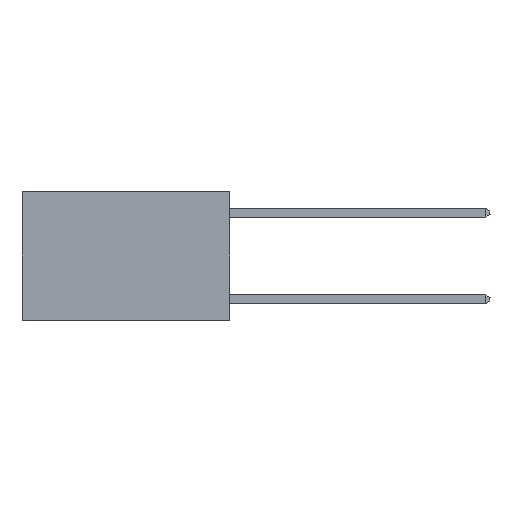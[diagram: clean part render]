
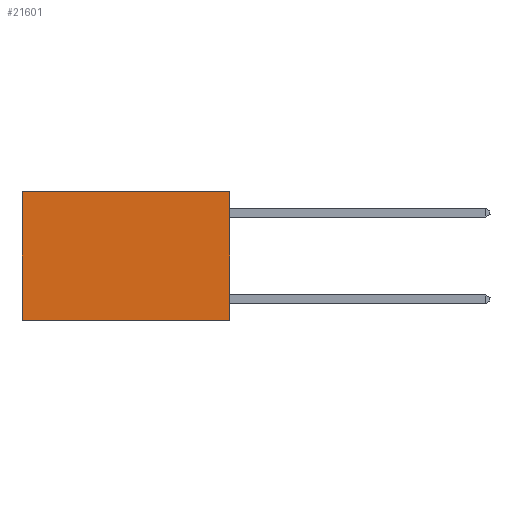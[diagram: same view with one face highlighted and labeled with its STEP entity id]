
A CAD part, left-side view. The second image highlights one B-rep face of the part: STEP entity #21601.
In plain terms, the highlighted planar face has unit normal (-1, 0, 0).
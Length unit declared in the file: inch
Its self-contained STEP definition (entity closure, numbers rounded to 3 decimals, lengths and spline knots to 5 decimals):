
#163 = VECTOR ( 'NONE', #21086, 39.37008 ) ;
#412 = ORIENTED_EDGE ( 'NONE', *, *, #11139, .T. ) ;
#1876 = EDGE_LOOP ( 'NONE', ( #2396, #12379, #10127, #412 ) ) ;
#2396 = ORIENTED_EDGE ( 'NONE', *, *, #17601, .T. ) ;
#2932 = LINE ( 'NONE', #8210, #163 ) ;
#3527 = CARTESIAN_POINT ( 'NONE',  ( 0.2625, 0., 0. ) ) ;
#5244 = CARTESIAN_POINT ( 'NONE',  ( 0.2625, 0., 0. ) ) ;
#5309 = CARTESIAN_POINT ( 'NONE',  ( 0.2625, 0.6, -0.37 ) ) ;
#5475 = PLANE ( 'NONE',  #11655 ) ;
#5821 = VERTEX_POINT ( 'NONE', #9431 ) ;
#8210 = CARTESIAN_POINT ( 'NONE',  ( 0.2625, 0., 0. ) ) ;
#8383 = CARTESIAN_POINT ( 'NONE',  ( 0.2625, 0., -0.37 ) ) ;
#9193 = DIRECTION ( 'NONE',  ( 1., 0., 0. ) ) ;
#9431 = CARTESIAN_POINT ( 'NONE',  ( 0.2625, 0.6, 0. ) ) ;
#10127 = ORIENTED_EDGE ( 'NONE', *, *, #12281, .F. ) ;
#11139 = EDGE_CURVE ( 'NONE', #19265, #5821, #2932, .T. ) ;
#11655 = AXIS2_PLACEMENT_3D ( 'NONE', #5244, #9193, #12565 ) ;
#12281 = EDGE_CURVE ( 'NONE', #19265, #16030, #19933, .T. ) ;
#12324 = VECTOR ( 'NONE', #15033, 39.37008 ) ;
#12379 = ORIENTED_EDGE ( 'NONE', *, *, #19711, .F. ) ;
#12565 = DIRECTION ( 'NONE',  ( 0., 0., -1. ) ) ;
#12941 = CARTESIAN_POINT ( 'NONE',  ( 0.2625, 0., -0.37 ) ) ;
#14922 = VECTOR ( 'NONE', #16267, 39.37008 ) ;
#15033 = DIRECTION ( 'NONE',  ( 0., 0., -1. ) ) ;
#15665 = CARTESIAN_POINT ( 'NONE',  ( 0.2625, 0.6, 0. ) ) ;
#16030 = VERTEX_POINT ( 'NONE', #8383 ) ;
#16267 = DIRECTION ( 'NONE',  ( 0., 1., 0. ) ) ;
#17601 = EDGE_CURVE ( 'NONE', #5821, #22495, #19488, .T. ) ;
#17857 = VECTOR ( 'NONE', #22932, 39.37008 ) ;
#19210 = CARTESIAN_POINT ( 'NONE',  ( 0.2625, 0., 0. ) ) ;
#19265 = VERTEX_POINT ( 'NONE', #19210 ) ;
#19488 = LINE ( 'NONE', #15665, #17857 ) ;
#19711 = EDGE_CURVE ( 'NONE', #16030, #22495, #20213, .T. ) ;
#19933 = LINE ( 'NONE', #3527, #12324 ) ;
#20213 = LINE ( 'NONE', #12941, #14922 ) ;
#21086 = DIRECTION ( 'NONE',  ( 0., 1., 0. ) ) ;
#21601 = ADVANCED_FACE ( 'NONE', ( #21633 ), #5475, .F. ) ;
#21633 = FACE_OUTER_BOUND ( 'NONE', #1876, .T. ) ;
#22495 = VERTEX_POINT ( 'NONE', #5309 ) ;
#22932 = DIRECTION ( 'NONE',  ( 0., 0., -1. ) ) ;
